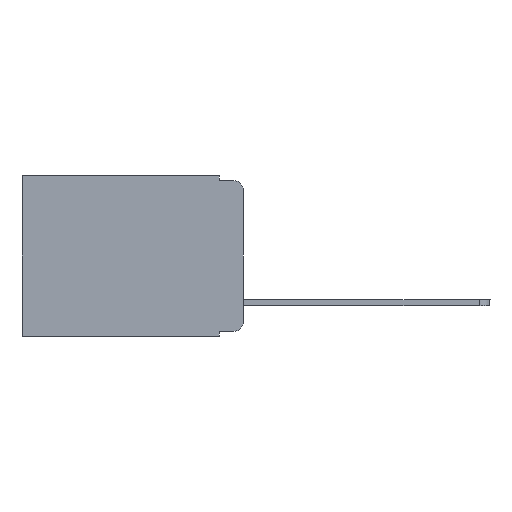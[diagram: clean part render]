
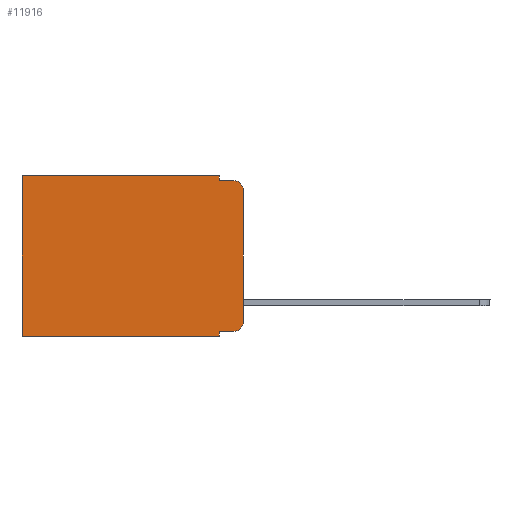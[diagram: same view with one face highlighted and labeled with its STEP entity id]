
A CAD part, left-side view. The second image highlights one B-rep face of the part: STEP entity #11916.
In plain terms, the highlighted planar face has unit normal (-1, 0, 0).
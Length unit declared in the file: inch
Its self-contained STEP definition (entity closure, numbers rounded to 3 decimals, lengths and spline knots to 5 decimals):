
#90 = VERTEX_POINT ( 'NONE', #9127 ) ;
#302 = VERTEX_POINT ( 'NONE', #8324 ) ;
#364 = CARTESIAN_POINT ( 'NONE',  ( 0.298, 0., 0. ) ) ;
#430 = LINE ( 'NONE', #2235, #8686 ) ;
#1029 = VECTOR ( 'NONE', #1719, 39.37008 ) ;
#1093 = CARTESIAN_POINT ( 'NONE',  ( 0.298, 0.051, -0.01 ) ) ;
#1130 = EDGE_CURVE ( 'NONE', #302, #4182, #15021, .T. ) ;
#1412 = LINE ( 'NONE', #10059, #8011 ) ;
#1542 = DIRECTION ( 'NONE',  ( 0., 0., -1. ) ) ;
#1707 = DIRECTION ( 'NONE',  ( 0., 0., -1. ) ) ;
#1719 = DIRECTION ( 'NONE',  ( 0., 1., 0. ) ) ;
#1982 = CARTESIAN_POINT ( 'NONE',  ( 0.298, 0.473, -0.343 ) ) ;
#2089 = VERTEX_POINT ( 'NONE', #1982 ) ;
#2204 = CARTESIAN_POINT ( 'NONE',  ( 0.298, 0.051, 0. ) ) ;
#2235 = CARTESIAN_POINT ( 'NONE',  ( 0.298, 0.051, -0.01 ) ) ;
#2351 = ORIENTED_EDGE ( 'NONE', *, *, #14736, .F. ) ;
#2657 = VECTOR ( 'NONE', #1707, 39.37008 ) ;
#2765 = VERTEX_POINT ( 'NONE', #5847 ) ;
#2892 = CIRCLE ( 'NONE', #10400, 0.02 ) ;
#3151 = DIRECTION ( 'NONE',  ( 0., 1., 0. ) ) ;
#3267 = VECTOR ( 'NONE', #13039, 39.37008 ) ;
#3735 = EDGE_CURVE ( 'NONE', #90, #4218, #2892, .T. ) ;
#3739 = CARTESIAN_POINT ( 'NONE',  ( 0.298, 0.02, -0.03 ) ) ;
#4182 = VERTEX_POINT ( 'NONE', #7993 ) ;
#4184 = LINE ( 'NONE', #8739, #1029 ) ;
#4218 = VERTEX_POINT ( 'NONE', #12648 ) ;
#4402 = EDGE_CURVE ( 'NONE', #90, #7408, #5254, .T. ) ;
#4869 = EDGE_LOOP ( 'NONE', ( #12432, #6087, #10546, #5928, #11386, #5739, #4940, #2351, #12818, #7285 ) ) ;
#4940 = ORIENTED_EDGE ( 'NONE', *, *, #9385, .F. ) ;
#5008 = CARTESIAN_POINT ( 'NONE',  ( 0.298, 0., -0.313 ) ) ;
#5254 = LINE ( 'NONE', #364, #5605 ) ;
#5605 = VECTOR ( 'NONE', #1542, 39.37008 ) ;
#5739 = ORIENTED_EDGE ( 'NONE', *, *, #10301, .T. ) ;
#5847 = CARTESIAN_POINT ( 'NONE',  ( 0.298, 0.473, 0. ) ) ;
#5902 = DIRECTION ( 'NONE',  ( 0., 0., -1. ) ) ;
#5928 = ORIENTED_EDGE ( 'NONE', *, *, #14555, .F. ) ;
#6087 = ORIENTED_EDGE ( 'NONE', *, *, #3735, .T. ) ;
#6101 = CARTESIAN_POINT ( 'NONE',  ( 0.298, 0.051, 0. ) ) ;
#6120 = LINE ( 'NONE', #6101, #2657 ) ;
#7034 = DIRECTION ( 'NONE',  ( 0., 0., -1. ) ) ;
#7285 = ORIENTED_EDGE ( 'NONE', *, *, #12863, .T. ) ;
#7408 = VERTEX_POINT ( 'NONE', #5008 ) ;
#7576 = FACE_OUTER_BOUND ( 'NONE', #4869, .T. ) ;
#7599 = CARTESIAN_POINT ( 'NONE',  ( 0.298, 0.02, -0.313 ) ) ;
#7827 = LINE ( 'NONE', #13232, #3267 ) ;
#7993 = CARTESIAN_POINT ( 'NONE',  ( 0.298, 0.02, -0.333 ) ) ;
#8011 = VECTOR ( 'NONE', #3151, 39.37008 ) ;
#8037 = LINE ( 'NONE', #8302, #13868 ) ;
#8302 = CARTESIAN_POINT ( 'NONE',  ( 0.298, 0.051, 0. ) ) ;
#8324 = CARTESIAN_POINT ( 'NONE',  ( 0.298, 0.051, -0.333 ) ) ;
#8626 = DIRECTION ( 'NONE',  ( 0., 0., -1. ) ) ;
#8686 = VECTOR ( 'NONE', #10412, 39.37008 ) ;
#8739 = CARTESIAN_POINT ( 'NONE',  ( 0.298, 0., 0. ) ) ;
#9037 = VERTEX_POINT ( 'NONE', #1093 ) ;
#9127 = CARTESIAN_POINT ( 'NONE',  ( 0.298, 0., -0.03 ) ) ;
#9385 = EDGE_CURVE ( 'NONE', #11790, #2089, #1412, .T. ) ;
#9513 = VERTEX_POINT ( 'NONE', #2204 ) ;
#9770 = CIRCLE ( 'NONE', #11746, 0.02 ) ;
#9830 = AXIS2_PLACEMENT_3D ( 'NONE', #11578, #12919, #7034 ) ;
#10059 = CARTESIAN_POINT ( 'NONE',  ( 0.298, 0., -0.343 ) ) ;
#10301 = EDGE_CURVE ( 'NONE', #2765, #2089, #7827, .T. ) ;
#10400 = AXIS2_PLACEMENT_3D ( 'NONE', #3739, #14260, #8626 ) ;
#10412 = DIRECTION ( 'NONE',  ( 0., -1., 0. ) ) ;
#10546 = ORIENTED_EDGE ( 'NONE', *, *, #11845, .F. ) ;
#10826 = EDGE_CURVE ( 'NONE', #9513, #2765, #4184, .T. ) ;
#11386 = ORIENTED_EDGE ( 'NONE', *, *, #10826, .T. ) ;
#11483 = PLANE ( 'NONE',  #9830 ) ;
#11578 = CARTESIAN_POINT ( 'NONE',  ( 0.298, 0., 0. ) ) ;
#11746 = AXIS2_PLACEMENT_3D ( 'NONE', #7599, #14532, #12288 ) ;
#11790 = VERTEX_POINT ( 'NONE', #13575 ) ;
#11845 = EDGE_CURVE ( 'NONE', #9037, #4218, #430, .T. ) ;
#11908 = VECTOR ( 'NONE', #13668, 39.37008 ) ;
#11916 = ADVANCED_FACE ( 'NONE', ( #7576 ), #11483, .F. ) ;
#12288 = DIRECTION ( 'NONE',  ( 0., 0., -1. ) ) ;
#12432 = ORIENTED_EDGE ( 'NONE', *, *, #4402, .F. ) ;
#12500 = CARTESIAN_POINT ( 'NONE',  ( 0.298, 0.051, -0.333 ) ) ;
#12648 = CARTESIAN_POINT ( 'NONE',  ( 0.298, 0.02, -0.01 ) ) ;
#12818 = ORIENTED_EDGE ( 'NONE', *, *, #1130, .T. ) ;
#12863 = EDGE_CURVE ( 'NONE', #4182, #7408, #9770, .T. ) ;
#12919 = DIRECTION ( 'NONE',  ( 1., 0., 0. ) ) ;
#13039 = DIRECTION ( 'NONE',  ( 0., 0., -1. ) ) ;
#13232 = CARTESIAN_POINT ( 'NONE',  ( 0.298, 0.473, 0. ) ) ;
#13575 = CARTESIAN_POINT ( 'NONE',  ( 0.298, 0.051, -0.343 ) ) ;
#13668 = DIRECTION ( 'NONE',  ( 0., -1., 0. ) ) ;
#13868 = VECTOR ( 'NONE', #5902, 39.37008 ) ;
#14260 = DIRECTION ( 'NONE',  ( -1., 0., 0. ) ) ;
#14532 = DIRECTION ( 'NONE',  ( -1., 0., 0. ) ) ;
#14555 = EDGE_CURVE ( 'NONE', #9513, #9037, #8037, .T. ) ;
#14736 = EDGE_CURVE ( 'NONE', #302, #11790, #6120, .T. ) ;
#15021 = LINE ( 'NONE', #12500, #11908 ) ;
